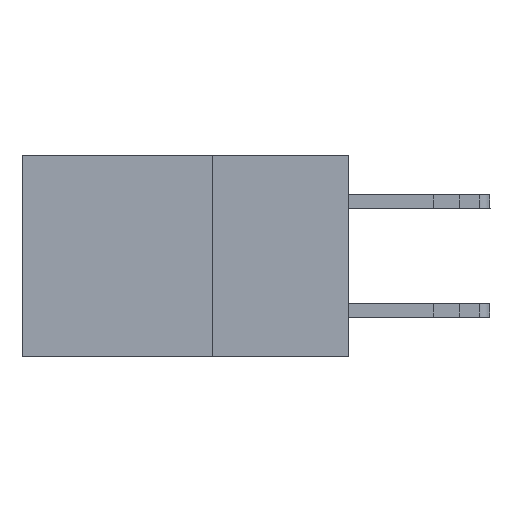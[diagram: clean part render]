
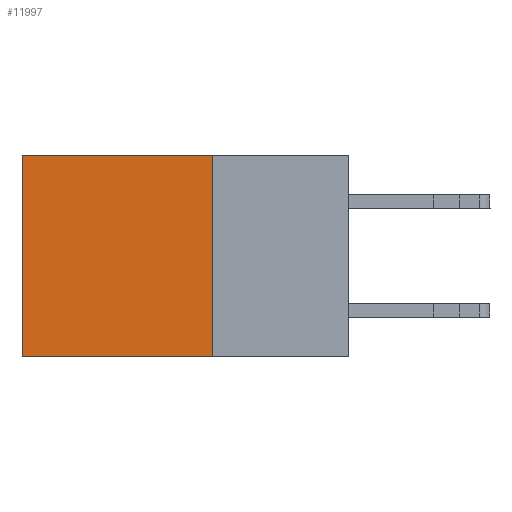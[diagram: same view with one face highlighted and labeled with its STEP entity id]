
A CAD part, left-side view. The second image highlights one B-rep face of the part: STEP entity #11997.
In plain terms, the highlighted planar face has unit normal (-1, 0, 0).
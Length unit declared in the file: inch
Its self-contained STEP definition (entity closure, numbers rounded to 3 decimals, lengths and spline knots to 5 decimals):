
#107 = AXIS2_PLACEMENT_3D ( 'NONE', #12914, #533, #21607 ) ;
#533 = DIRECTION ( 'NONE',  ( 1., 0., 0. ) ) ;
#1069 = VERTEX_POINT ( 'NONE', #19889 ) ;
#1954 = CARTESIAN_POINT ( 'NONE',  ( 0.2615, 0.25, -0.37 ) ) ;
#4444 = EDGE_CURVE ( 'NONE', #21009, #5092, #6864, .T. ) ;
#5092 = VERTEX_POINT ( 'NONE', #15990 ) ;
#5233 = VECTOR ( 'NONE', #16638, 39.37008 ) ;
#6225 = ORIENTED_EDGE ( 'NONE', *, *, #15967, .F. ) ;
#6583 = VERTEX_POINT ( 'NONE', #9447 ) ;
#6864 = LINE ( 'NONE', #20996, #19769 ) ;
#7211 = ORIENTED_EDGE ( 'NONE', *, *, #16432, .T. ) ;
#7346 = DIRECTION ( 'NONE',  ( 0., 0., -1. ) ) ;
#9447 = CARTESIAN_POINT ( 'NONE',  ( 0.2615, 0.6, 0. ) ) ;
#10733 = ORIENTED_EDGE ( 'NONE', *, *, #11609, .T. ) ;
#11609 = EDGE_CURVE ( 'NONE', #1069, #6583, #14681, .T. ) ;
#11997 = ADVANCED_FACE ( 'NONE', ( #16500 ), #19872, .F. ) ;
#12712 = CARTESIAN_POINT ( 'NONE',  ( 0.2615, 0.25, 0. ) ) ;
#12914 = CARTESIAN_POINT ( 'NONE',  ( 0.2615, 0.25, -0.37 ) ) ;
#14196 = LINE ( 'NONE', #19529, #19977 ) ;
#14681 = LINE ( 'NONE', #12712, #5233 ) ;
#15824 = ORIENTED_EDGE ( 'NONE', *, *, #4444, .F. ) ;
#15904 = EDGE_LOOP ( 'NONE', ( #7211, #15824, #6225, #10733 ) ) ;
#15967 = EDGE_CURVE ( 'NONE', #1069, #21009, #14196, .T. ) ;
#15982 = LINE ( 'NONE', #19585, #20381 ) ;
#15990 = CARTESIAN_POINT ( 'NONE',  ( 0.2615, 0.6, -0.37 ) ) ;
#16432 = EDGE_CURVE ( 'NONE', #6583, #5092, #15982, .T. ) ;
#16500 = FACE_OUTER_BOUND ( 'NONE', #15904, .T. ) ;
#16638 = DIRECTION ( 'NONE',  ( 0., 1., 0. ) ) ;
#19397 = DIRECTION ( 'NONE',  ( 0., 1., 0. ) ) ;
#19529 = CARTESIAN_POINT ( 'NONE',  ( 0.2615, 0.25, -0.37 ) ) ;
#19585 = CARTESIAN_POINT ( 'NONE',  ( 0.2615, 0.6, -0.37 ) ) ;
#19769 = VECTOR ( 'NONE', #19397, 39.37008 ) ;
#19872 = PLANE ( 'NONE',  #107 ) ;
#19889 = CARTESIAN_POINT ( 'NONE',  ( 0.2615, 0.25, 0. ) ) ;
#19977 = VECTOR ( 'NONE', #7346, 39.37008 ) ;
#20381 = VECTOR ( 'NONE', #21551, 39.37008 ) ;
#20996 = CARTESIAN_POINT ( 'NONE',  ( 0.2615, 0.25, -0.37 ) ) ;
#21009 = VERTEX_POINT ( 'NONE', #1954 ) ;
#21551 = DIRECTION ( 'NONE',  ( 0., 0., -1. ) ) ;
#21607 = DIRECTION ( 'NONE',  ( 0., 0., -1. ) ) ;
